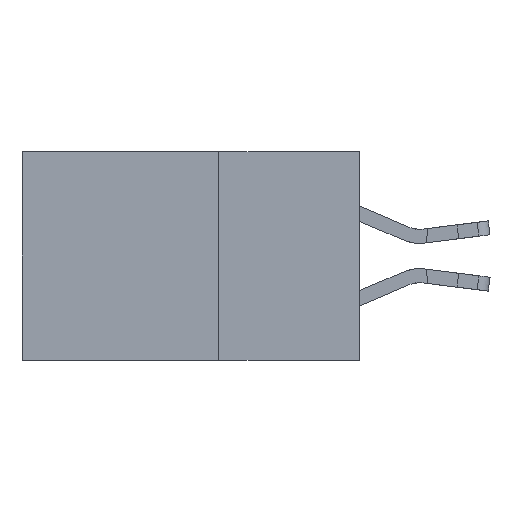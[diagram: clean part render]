
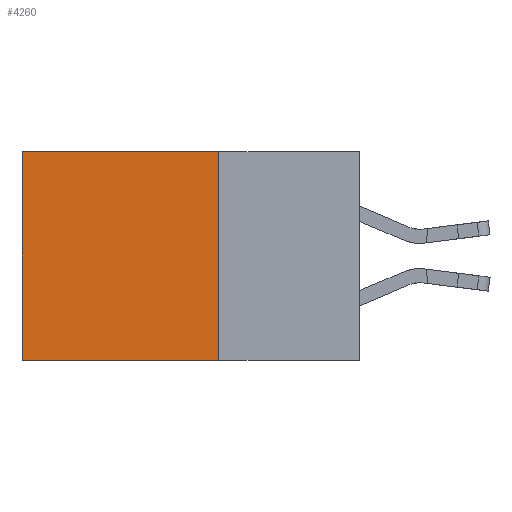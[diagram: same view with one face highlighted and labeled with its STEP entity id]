
A CAD part, left-side view. The second image highlights one B-rep face of the part: STEP entity #4260.
In plain terms, the highlighted planar face has unit normal (-1, 0, 0).
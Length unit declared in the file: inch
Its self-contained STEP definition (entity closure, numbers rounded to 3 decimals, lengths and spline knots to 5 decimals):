
#32 = CARTESIAN_POINT ( 'NONE',  ( 0.2875, 0.25, 0. ) ) ;
#504 = EDGE_CURVE ( 'NONE', #19453, #3119, #18569, .T. ) ;
#1035 = ORIENTED_EDGE ( 'NONE', *, *, #10718, .T. ) ;
#1182 = AXIS2_PLACEMENT_3D ( 'NONE', #19089, #12785, #1433 ) ;
#1206 = VECTOR ( 'NONE', #3493, 39.37008 ) ;
#1433 = DIRECTION ( 'NONE',  ( 0., 0., -1. ) ) ;
#1840 = CARTESIAN_POINT ( 'NONE',  ( 0.2875, 0.25, 0. ) ) ;
#2009 = LINE ( 'NONE', #14144, #20156 ) ;
#3119 = VERTEX_POINT ( 'NONE', #18452 ) ;
#3493 = DIRECTION ( 'NONE',  ( 0., 0., -1. ) ) ;
#3663 = ORIENTED_EDGE ( 'NONE', *, *, #20383, .T. ) ;
#4260 = ADVANCED_FACE ( 'NONE', ( #12366 ), #10921, .F. ) ;
#4585 = CARTESIAN_POINT ( 'NONE',  ( 0.2875, 0.6, 0. ) ) ;
#6160 = LINE ( 'NONE', #20407, #6663 ) ;
#6646 = VERTEX_POINT ( 'NONE', #17410 ) ;
#6663 = VECTOR ( 'NONE', #17268, 39.37008 ) ;
#8101 = ORIENTED_EDGE ( 'NONE', *, *, #13799, .F. ) ;
#8436 = LINE ( 'NONE', #32, #16509 ) ;
#10299 = DIRECTION ( 'NONE',  ( 0., 1., 0. ) ) ;
#10718 = EDGE_CURVE ( 'NONE', #13831, #6646, #2009, .T. ) ;
#10921 = PLANE ( 'NONE',  #1182 ) ;
#12168 = EDGE_LOOP ( 'NONE', ( #1035, #8101, #13150, #3663 ) ) ;
#12178 = CARTESIAN_POINT ( 'NONE',  ( 0.2875, 0.25, 0. ) ) ;
#12366 = FACE_OUTER_BOUND ( 'NONE', #12168, .T. ) ;
#12615 = DIRECTION ( 'NONE',  ( 0., 0., -1. ) ) ;
#12785 = DIRECTION ( 'NONE',  ( 1., 0., 0. ) ) ;
#13150 = ORIENTED_EDGE ( 'NONE', *, *, #504, .F. ) ;
#13799 = EDGE_CURVE ( 'NONE', #3119, #6646, #6160, .T. ) ;
#13831 = VERTEX_POINT ( 'NONE', #4585 ) ;
#14144 = CARTESIAN_POINT ( 'NONE',  ( 0.2875, 0.6, 0. ) ) ;
#16509 = VECTOR ( 'NONE', #10299, 39.37008 ) ;
#17268 = DIRECTION ( 'NONE',  ( 0., 1., 0. ) ) ;
#17410 = CARTESIAN_POINT ( 'NONE',  ( 0.2875, 0.6, -0.37 ) ) ;
#18452 = CARTESIAN_POINT ( 'NONE',  ( 0.2875, 0.25, -0.37 ) ) ;
#18569 = LINE ( 'NONE', #1840, #1206 ) ;
#19089 = CARTESIAN_POINT ( 'NONE',  ( 0.2875, 0.25, 0. ) ) ;
#19453 = VERTEX_POINT ( 'NONE', #12178 ) ;
#20156 = VECTOR ( 'NONE', #12615, 39.37008 ) ;
#20383 = EDGE_CURVE ( 'NONE', #19453, #13831, #8436, .T. ) ;
#20407 = CARTESIAN_POINT ( 'NONE',  ( 0.2875, 0.25, -0.37 ) ) ;
